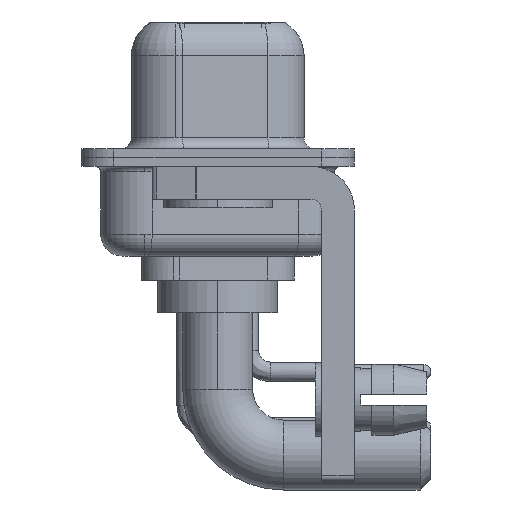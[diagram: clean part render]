
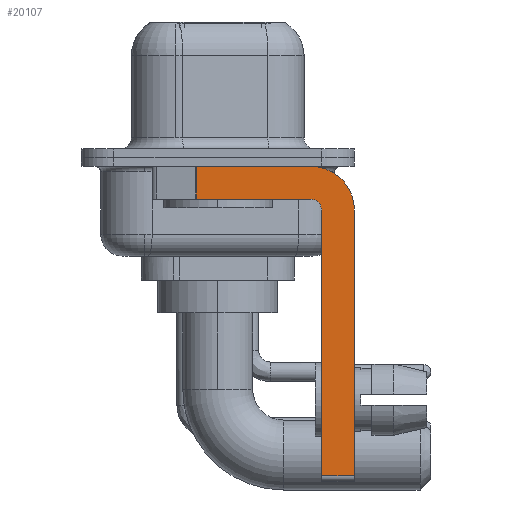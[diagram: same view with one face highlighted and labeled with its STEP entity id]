
A CAD part, left-side view. The second image highlights one B-rep face of the part: STEP entity #20107.
In plain terms, the highlighted planar face has unit normal (-1, 0, 0).
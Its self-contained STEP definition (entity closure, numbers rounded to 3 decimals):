
#379 = CIRCLE ( 'NONE', #4004, 0.5 ) ;
#651 = CARTESIAN_POINT ( 'NONE',  ( -2.9, -4.25, -1.9 ) ) ;
#859 = AXIS2_PLACEMENT_3D ( 'NONE', #8781, #1793, #8886 ) ;
#1447 = EDGE_LOOP ( 'NONE', ( #4970, #18887, #11136, #20419, #8087, #2436, #8503, #21950 ) ) ;
#1545 = LINE ( 'NONE', #8767, #4514 ) ;
#1556 = EDGE_CURVE ( 'NONE', #12156, #8822, #19158, .T. ) ;
#1793 = DIRECTION ( 'NONE',  ( 1., 0., 0. ) ) ;
#2008 = PLANE ( 'NONE',  #859 ) ;
#2404 = EDGE_CURVE ( 'NONE', #11461, #10501, #379, .T. ) ;
#2436 = ORIENTED_EDGE ( 'NONE', *, *, #20998, .T. ) ;
#2874 = CARTESIAN_POINT ( 'NONE',  ( -2.9, -6.25, -14.55 ) ) ;
#3028 = VECTOR ( 'NONE', #3403, 1000. ) ;
#3335 = DIRECTION ( 'NONE',  ( 0., 0., -1. ) ) ;
#3403 = DIRECTION ( 'NONE',  ( 0., 0., 1. ) ) ;
#4004 = AXIS2_PLACEMENT_3D ( 'NONE', #7929, #21889, #6306 ) ;
#4514 = VECTOR ( 'NONE', #5100, 1000. ) ;
#4970 = ORIENTED_EDGE ( 'NONE', *, *, #7393, .F. ) ;
#5100 = DIRECTION ( 'NONE',  ( 0., 0., -1. ) ) ;
#5945 = DIRECTION ( 'NONE',  ( 0., 0., -1. ) ) ;
#6002 = CARTESIAN_POINT ( 'NONE',  ( -2.9, -4.25, -0.4 ) ) ;
#6113 = EDGE_CURVE ( 'NONE', #11411, #12741, #13346, .T. ) ;
#6306 = DIRECTION ( 'NONE',  ( 0., 0., 1. ) ) ;
#6414 = EDGE_CURVE ( 'NONE', #7850, #11461, #17380, .T. ) ;
#6609 = VECTOR ( 'NONE', #7117, 1000. ) ;
#6729 = CARTESIAN_POINT ( 'NONE',  ( -2.9, -4.25, -14.55 ) ) ;
#7117 = DIRECTION ( 'NONE',  ( 0., -1., 0. ) ) ;
#7393 = EDGE_CURVE ( 'NONE', #12156, #11411, #15814, .T. ) ;
#7397 = VECTOR ( 'NONE', #17256, 1000. ) ;
#7496 = AXIS2_PLACEMENT_3D ( 'NONE', #12811, #18199, #5945 ) ;
#7777 = CARTESIAN_POINT ( 'NONE',  ( -2.9, -4.25, -1.9 ) ) ;
#7850 = VERTEX_POINT ( 'NONE', #8688 ) ;
#7929 = CARTESIAN_POINT ( 'NONE',  ( -2.9, -4.25, -2.4 ) ) ;
#8087 = ORIENTED_EDGE ( 'NONE', *, *, #6414, .F. ) ;
#8503 = ORIENTED_EDGE ( 'NONE', *, *, #21612, .F. ) ;
#8688 = CARTESIAN_POINT ( 'NONE',  ( -2.9, -4.75, -14.55 ) ) ;
#8767 = CARTESIAN_POINT ( 'NONE',  ( -2.9, -6.25, -2.4 ) ) ;
#8781 = CARTESIAN_POINT ( 'NONE',  ( -2.9, -4.25, -2.4 ) ) ;
#8822 = VERTEX_POINT ( 'NONE', #15801 ) ;
#8886 = DIRECTION ( 'NONE',  ( 0., 0., -1. ) ) ;
#10501 = VERTEX_POINT ( 'NONE', #7777 ) ;
#11136 = ORIENTED_EDGE ( 'NONE', *, *, #16223, .F. ) ;
#11155 = CARTESIAN_POINT ( 'NONE',  ( -2.9, -4.75, -2.4 ) ) ;
#11323 = VECTOR ( 'NONE', #3335, 1000. ) ;
#11411 = VERTEX_POINT ( 'NONE', #6002 ) ;
#11461 = VERTEX_POINT ( 'NONE', #11155 ) ;
#11943 = CARTESIAN_POINT ( 'NONE',  ( -2.9, -6.25, -2.4 ) ) ;
#12156 = VERTEX_POINT ( 'NONE', #19444 ) ;
#12741 = VERTEX_POINT ( 'NONE', #11943 ) ;
#12811 = CARTESIAN_POINT ( 'NONE',  ( -2.9, -4.25, -2.4 ) ) ;
#13346 = CIRCLE ( 'NONE', #7496, 2. ) ;
#13420 = VERTEX_POINT ( 'NONE', #2874 ) ;
#13792 = VECTOR ( 'NONE', #21713, 1000. ) ;
#14213 = CARTESIAN_POINT ( 'NONE',  ( -2.9, 3., -0.4 ) ) ;
#15801 = CARTESIAN_POINT ( 'NONE',  ( -2.9, 0.978, -1.9 ) ) ;
#15814 = LINE ( 'NONE', #14213, #6609 ) ;
#16223 = EDGE_CURVE ( 'NONE', #10501, #8822, #16331, .T. ) ;
#16331 = LINE ( 'NONE', #651, #13792 ) ;
#16809 = LINE ( 'NONE', #6729, #7397 ) ;
#17256 = DIRECTION ( 'NONE',  ( 0., -1., 0. ) ) ;
#17362 = FACE_OUTER_BOUND ( 'NONE', #1447, .T. ) ;
#17380 = LINE ( 'NONE', #20935, #3028 ) ;
#18199 = DIRECTION ( 'NONE',  ( 1., 0., 0. ) ) ;
#18887 = ORIENTED_EDGE ( 'NONE', *, *, #1556, .T. ) ;
#19158 = LINE ( 'NONE', #22582, #11323 ) ;
#19444 = CARTESIAN_POINT ( 'NONE',  ( -2.9, 0.978, -0.4 ) ) ;
#20107 = ADVANCED_FACE ( 'NONE', ( #17362 ), #2008, .F. ) ;
#20419 = ORIENTED_EDGE ( 'NONE', *, *, #2404, .F. ) ;
#20935 = CARTESIAN_POINT ( 'NONE',  ( -2.9, -4.75, -14.8 ) ) ;
#20998 = EDGE_CURVE ( 'NONE', #7850, #13420, #16809, .T. ) ;
#21612 = EDGE_CURVE ( 'NONE', #12741, #13420, #1545, .T. ) ;
#21713 = DIRECTION ( 'NONE',  ( 0., 1., 0. ) ) ;
#21889 = DIRECTION ( 'NONE',  ( -1., 0., 0. ) ) ;
#21950 = ORIENTED_EDGE ( 'NONE', *, *, #6113, .F. ) ;
#22582 = CARTESIAN_POINT ( 'NONE',  ( -2.9, 0.978, -1.9 ) ) ;
